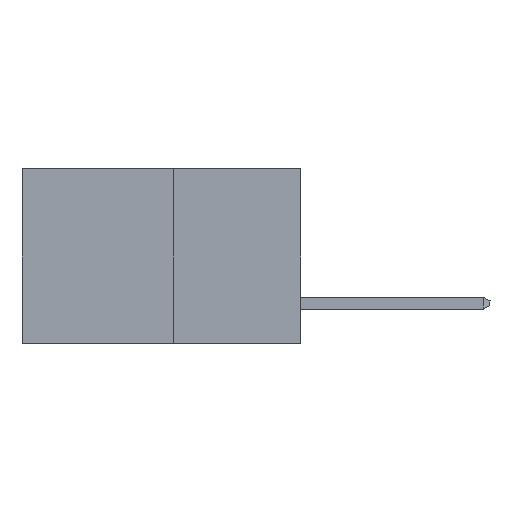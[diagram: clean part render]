
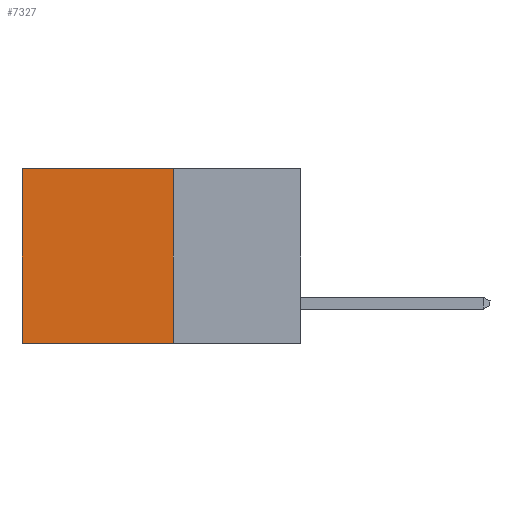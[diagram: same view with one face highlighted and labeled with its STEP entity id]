
A CAD part, left-side view. The second image highlights one B-rep face of the part: STEP entity #7327.
In plain terms, the highlighted planar face has unit normal (-1, 0, 0).
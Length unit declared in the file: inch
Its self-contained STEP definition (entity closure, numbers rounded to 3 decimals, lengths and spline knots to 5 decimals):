
#778 = DIRECTION ( 'NONE',  ( 0., 0., -1. ) ) ;
#1194 = ORIENTED_EDGE ( 'NONE', *, *, #6029, .F. ) ;
#2280 = LINE ( 'NONE', #11491, #12220 ) ;
#2528 = LINE ( 'NONE', #8875, #12440 ) ;
#3792 = CARTESIAN_POINT ( 'NONE',  ( 0.277, 0.27, 0. ) ) ;
#4054 = VERTEX_POINT ( 'NONE', #3792 ) ;
#4620 = ORIENTED_EDGE ( 'NONE', *, *, #12329, .T. ) ;
#4784 = EDGE_CURVE ( 'NONE', #7332, #8137, #2280, .T. ) ;
#4937 = DIRECTION ( 'NONE',  ( 1., 0., 0. ) ) ;
#5922 = CARTESIAN_POINT ( 'NONE',  ( 0.277, 0.59, 0. ) ) ;
#6029 = EDGE_CURVE ( 'NONE', #4054, #7332, #10300, .T. ) ;
#6231 = DIRECTION ( 'NONE',  ( 0., 0., -1. ) ) ;
#6282 = CARTESIAN_POINT ( 'NONE',  ( 0.277, 0.27, -0.37 ) ) ;
#6311 = DIRECTION ( 'NONE',  ( 0., 1., 0. ) ) ;
#6445 = CARTESIAN_POINT ( 'NONE',  ( 0.277, 0.59, -0.37 ) ) ;
#7138 = CARTESIAN_POINT ( 'NONE',  ( 0.277, 0.59, -0.37 ) ) ;
#7184 = ORIENTED_EDGE ( 'NONE', *, *, #9807, .T. ) ;
#7327 = ADVANCED_FACE ( 'NONE', ( #13333 ), #12317, .F. ) ;
#7332 = VERTEX_POINT ( 'NONE', #9851 ) ;
#7883 = VERTEX_POINT ( 'NONE', #5922 ) ;
#8137 = VERTEX_POINT ( 'NONE', #6445 ) ;
#8875 = CARTESIAN_POINT ( 'NONE',  ( 0.277, 0.27, 0. ) ) ;
#9331 = LINE ( 'NONE', #7138, #12166 ) ;
#9807 = EDGE_CURVE ( 'NONE', #7883, #8137, #9331, .T. ) ;
#9851 = CARTESIAN_POINT ( 'NONE',  ( 0.277, 0.27, -0.37 ) ) ;
#10300 = LINE ( 'NONE', #6282, #15855 ) ;
#11198 = EDGE_LOOP ( 'NONE', ( #7184, #13620, #1194, #4620 ) ) ;
#11491 = CARTESIAN_POINT ( 'NONE',  ( 0.277, 0.27, -0.37 ) ) ;
#11515 = DIRECTION ( 'NONE',  ( 0., 1., 0. ) ) ;
#12166 = VECTOR ( 'NONE', #778, 39.37008 ) ;
#12220 = VECTOR ( 'NONE', #11515, 39.37008 ) ;
#12317 = PLANE ( 'NONE',  #14667 ) ;
#12329 = EDGE_CURVE ( 'NONE', #4054, #7883, #2528, .T. ) ;
#12440 = VECTOR ( 'NONE', #6311, 39.37008 ) ;
#13333 = FACE_OUTER_BOUND ( 'NONE', #11198, .T. ) ;
#13449 = CARTESIAN_POINT ( 'NONE',  ( 0.277, 0.27, -0.37 ) ) ;
#13504 = DIRECTION ( 'NONE',  ( 0., 0., -1. ) ) ;
#13620 = ORIENTED_EDGE ( 'NONE', *, *, #4784, .F. ) ;
#14667 = AXIS2_PLACEMENT_3D ( 'NONE', #13449, #4937, #13504 ) ;
#15855 = VECTOR ( 'NONE', #6231, 39.37008 ) ;
